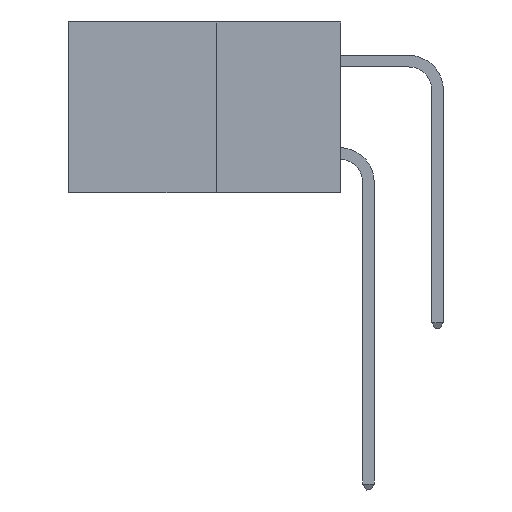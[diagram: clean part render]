
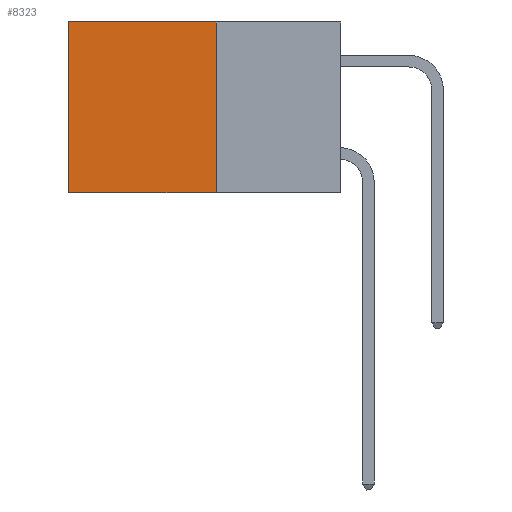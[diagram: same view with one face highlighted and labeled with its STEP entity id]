
A CAD part, left-side view. The second image highlights one B-rep face of the part: STEP entity #8323.
In plain terms, the highlighted planar face has unit normal (-1, 0, 0).
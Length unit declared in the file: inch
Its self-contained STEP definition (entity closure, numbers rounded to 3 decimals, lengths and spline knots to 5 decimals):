
#163 = DIRECTION ( 'NONE',  ( 0., 0., -1. ) ) ;
#209 = DIRECTION ( 'NONE',  ( 0., 0., -1. ) ) ;
#231 = VERTEX_POINT ( 'NONE', #5398 ) ;
#366 = VERTEX_POINT ( 'NONE', #9947 ) ;
#405 = EDGE_CURVE ( 'NONE', #4882, #366, #6313, .T. ) ;
#774 = VECTOR ( 'NONE', #10199, 39.37008 ) ;
#1050 = LINE ( 'NONE', #2051, #774 ) ;
#1131 = ORIENTED_EDGE ( 'NONE', *, *, #8678, .F. ) ;
#1318 = VECTOR ( 'NONE', #9931, 39.37008 ) ;
#1669 = CARTESIAN_POINT ( 'NONE',  ( 0.277, 0.59, 0. ) ) ;
#2051 = CARTESIAN_POINT ( 'NONE',  ( 0.277, 0.27, 0. ) ) ;
#2843 = CARTESIAN_POINT ( 'NONE',  ( 0.277, 0.27, -0.37 ) ) ;
#3590 = CARTESIAN_POINT ( 'NONE',  ( 0.277, 0.27, -0.37 ) ) ;
#3891 = CARTESIAN_POINT ( 'NONE',  ( 0.277, 0.27, -0.37 ) ) ;
#3961 = CARTESIAN_POINT ( 'NONE',  ( 0.277, 0.27, -0.37 ) ) ;
#4775 = ORIENTED_EDGE ( 'NONE', *, *, #9877, .T. ) ;
#4811 = DIRECTION ( 'NONE',  ( 1., 0., 0. ) ) ;
#4882 = VERTEX_POINT ( 'NONE', #3891 ) ;
#5304 = FACE_OUTER_BOUND ( 'NONE', #6718, .T. ) ;
#5398 = CARTESIAN_POINT ( 'NONE',  ( 0.277, 0.27, 0. ) ) ;
#6068 = LINE ( 'NONE', #3590, #9836 ) ;
#6119 = ORIENTED_EDGE ( 'NONE', *, *, #9388, .T. ) ;
#6313 = LINE ( 'NONE', #2843, #1318 ) ;
#6718 = EDGE_LOOP ( 'NONE', ( #4775, #7291, #1131, #6119 ) ) ;
#7277 = VERTEX_POINT ( 'NONE', #1669 ) ;
#7291 = ORIENTED_EDGE ( 'NONE', *, *, #405, .F. ) ;
#7743 = CARTESIAN_POINT ( 'NONE',  ( 0.277, 0.59, -0.37 ) ) ;
#7992 = AXIS2_PLACEMENT_3D ( 'NONE', #3961, #4811, #10453 ) ;
#8323 = ADVANCED_FACE ( 'NONE', ( #5304 ), #8836, .F. ) ;
#8678 = EDGE_CURVE ( 'NONE', #231, #4882, #6068, .T. ) ;
#8810 = VECTOR ( 'NONE', #209, 39.37008 ) ;
#8836 = PLANE ( 'NONE',  #7992 ) ;
#9063 = LINE ( 'NONE', #7743, #8810 ) ;
#9388 = EDGE_CURVE ( 'NONE', #231, #7277, #1050, .T. ) ;
#9836 = VECTOR ( 'NONE', #163, 39.37008 ) ;
#9877 = EDGE_CURVE ( 'NONE', #7277, #366, #9063, .T. ) ;
#9931 = DIRECTION ( 'NONE',  ( 0., 1., 0. ) ) ;
#9947 = CARTESIAN_POINT ( 'NONE',  ( 0.277, 0.59, -0.37 ) ) ;
#10199 = DIRECTION ( 'NONE',  ( 0., 1., 0. ) ) ;
#10453 = DIRECTION ( 'NONE',  ( 0., 0., -1. ) ) ;
